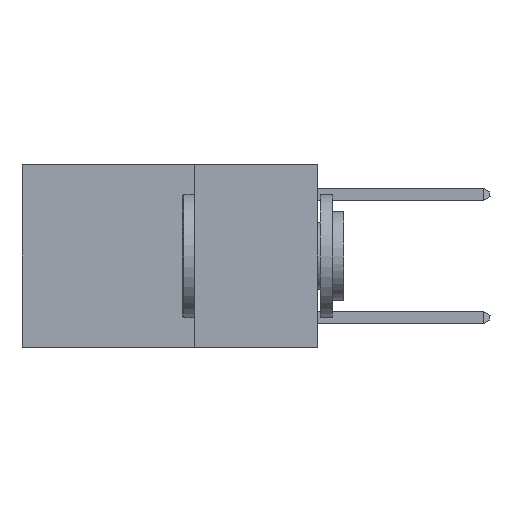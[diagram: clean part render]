
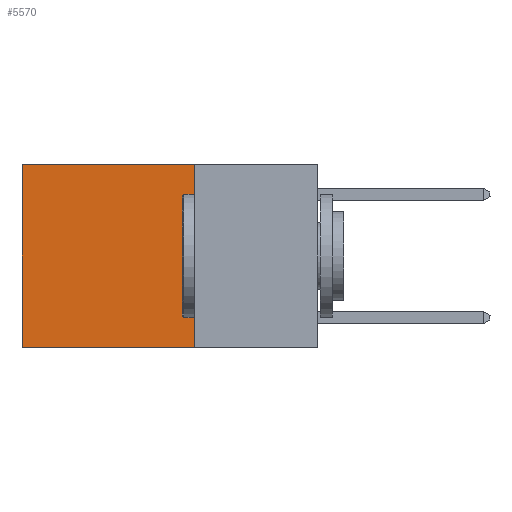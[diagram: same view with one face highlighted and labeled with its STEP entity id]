
A CAD part, left-side view. The second image highlights one B-rep face of the part: STEP entity #5570.
In plain terms, the highlighted planar face has unit normal (-1, 0, 0).
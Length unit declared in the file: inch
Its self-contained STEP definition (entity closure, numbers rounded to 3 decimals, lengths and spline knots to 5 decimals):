
#1695 = DIRECTION ( 'NONE',  ( 0., 1., 0. ) ) ;
#1813 = CARTESIAN_POINT ( 'NONE',  ( 0.2625, 0.25, 0. ) ) ;
#2387 = PLANE ( 'NONE',  #23795 ) ;
#2497 = VECTOR ( 'NONE', #1695, 39.37008 ) ;
#2573 = VERTEX_POINT ( 'NONE', #13190 ) ;
#4295 = DIRECTION ( 'NONE',  ( 0., 1., 0. ) ) ;
#4393 = ORIENTED_EDGE ( 'NONE', *, *, #18221, .T. ) ;
#4415 = EDGE_CURVE ( 'NONE', #18789, #2573, #11114, .T. ) ;
#5533 = VECTOR ( 'NONE', #4295, 39.37008 ) ;
#5570 = ADVANCED_FACE ( 'NONE', ( #7816 ), #2387, .F. ) ;
#5769 = CARTESIAN_POINT ( 'NONE',  ( 0.2625, 0.6, -0.37 ) ) ;
#5879 = ORIENTED_EDGE ( 'NONE', *, *, #7349, .F. ) ;
#6146 = VECTOR ( 'NONE', #21570, 39.37008 ) ;
#7349 = EDGE_CURVE ( 'NONE', #10475, #13286, #22440, .T. ) ;
#7816 = FACE_OUTER_BOUND ( 'NONE', #12192, .T. ) ;
#7934 = CARTESIAN_POINT ( 'NONE',  ( 0.2625, 0.25, 0. ) ) ;
#8237 = LINE ( 'NONE', #22887, #11551 ) ;
#9615 = CARTESIAN_POINT ( 'NONE',  ( 0.2625, 0.25, -0.37 ) ) ;
#9751 = DIRECTION ( 'NONE',  ( 1., 0., 0. ) ) ;
#10475 = VERTEX_POINT ( 'NONE', #14315 ) ;
#11114 = LINE ( 'NONE', #1813, #2497 ) ;
#11551 = VECTOR ( 'NONE', #12232, 39.37008 ) ;
#12192 = EDGE_LOOP ( 'NONE', ( #4393, #5879, #23136, #14778 ) ) ;
#12232 = DIRECTION ( 'NONE',  ( 0., 0., -1. ) ) ;
#12376 = LINE ( 'NONE', #17464, #6146 ) ;
#13190 = CARTESIAN_POINT ( 'NONE',  ( 0.2625, 0.6, 0. ) ) ;
#13286 = VERTEX_POINT ( 'NONE', #5769 ) ;
#14315 = CARTESIAN_POINT ( 'NONE',  ( 0.2625, 0.25, -0.37 ) ) ;
#14407 = CARTESIAN_POINT ( 'NONE',  ( 0.2625, 0.25, 0. ) ) ;
#14778 = ORIENTED_EDGE ( 'NONE', *, *, #4415, .T. ) ;
#17129 = DIRECTION ( 'NONE',  ( 0., 0., -1. ) ) ;
#17464 = CARTESIAN_POINT ( 'NONE',  ( 0.2625, 0.6, 0. ) ) ;
#18221 = EDGE_CURVE ( 'NONE', #2573, #13286, #12376, .T. ) ;
#18752 = EDGE_CURVE ( 'NONE', #18789, #10475, #8237, .T. ) ;
#18789 = VERTEX_POINT ( 'NONE', #14407 ) ;
#21570 = DIRECTION ( 'NONE',  ( 0., 0., -1. ) ) ;
#22440 = LINE ( 'NONE', #9615, #5533 ) ;
#22887 = CARTESIAN_POINT ( 'NONE',  ( 0.2625, 0.25, 0. ) ) ;
#23136 = ORIENTED_EDGE ( 'NONE', *, *, #18752, .F. ) ;
#23795 = AXIS2_PLACEMENT_3D ( 'NONE', #7934, #9751, #17129 ) ;
